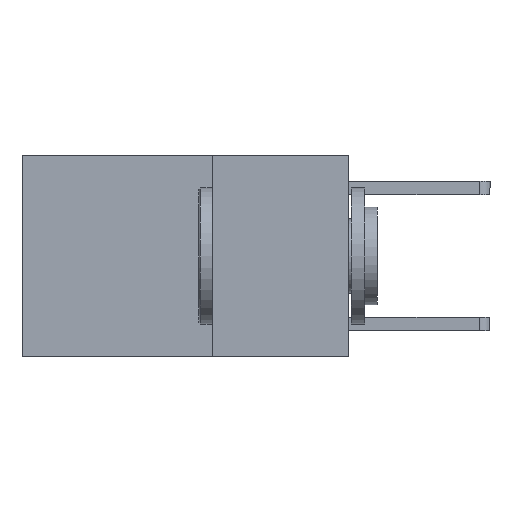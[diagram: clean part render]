
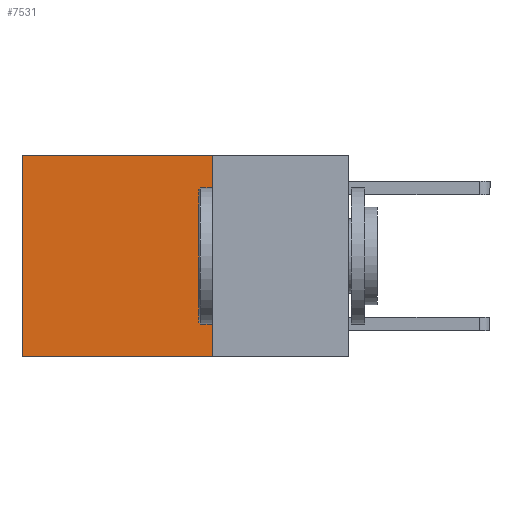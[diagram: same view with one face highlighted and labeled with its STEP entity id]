
A CAD part, left-side view. The second image highlights one B-rep face of the part: STEP entity #7531.
In plain terms, the highlighted planar face has unit normal (-1, 0, 0).
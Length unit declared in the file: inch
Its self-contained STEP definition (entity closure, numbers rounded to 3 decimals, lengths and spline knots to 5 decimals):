
#411 = EDGE_LOOP ( 'NONE', ( #4939, #6065, #1197, #7677 ) ) ;
#567 = PLANE ( 'NONE',  #1010 ) ;
#927 = VERTEX_POINT ( 'NONE', #7669 ) ;
#1010 = AXIS2_PLACEMENT_3D ( 'NONE', #4209, #9289, #8355 ) ;
#1098 = LINE ( 'NONE', #1873, #3606 ) ;
#1111 = VECTOR ( 'NONE', #6720, 39.37008 ) ;
#1197 = ORIENTED_EDGE ( 'NONE', *, *, #2684, .F. ) ;
#1653 = VERTEX_POINT ( 'NONE', #7351 ) ;
#1873 = CARTESIAN_POINT ( 'NONE',  ( 0.2625, 0.25, 0. ) ) ;
#1903 = VERTEX_POINT ( 'NONE', #5419 ) ;
#1950 = VECTOR ( 'NONE', #5726, 39.37008 ) ;
#2103 = CARTESIAN_POINT ( 'NONE',  ( 0.2625, 0.25, -0.37 ) ) ;
#2136 = EDGE_CURVE ( 'NONE', #1653, #927, #4411, .T. ) ;
#2684 = EDGE_CURVE ( 'NONE', #5913, #1903, #6620, .T. ) ;
#3606 = VECTOR ( 'NONE', #7428, 39.37008 ) ;
#4209 = CARTESIAN_POINT ( 'NONE',  ( 0.2625, 0.25, 0. ) ) ;
#4312 = CARTESIAN_POINT ( 'NONE',  ( 0.2625, 0.6, 0. ) ) ;
#4411 = LINE ( 'NONE', #4312, #8078 ) ;
#4884 = LINE ( 'NONE', #2103, #1950 ) ;
#4939 = ORIENTED_EDGE ( 'NONE', *, *, #2136, .T. ) ;
#5419 = CARTESIAN_POINT ( 'NONE',  ( 0.2625, 0.25, -0.37 ) ) ;
#5726 = DIRECTION ( 'NONE',  ( 0., 1., 0. ) ) ;
#5913 = VERTEX_POINT ( 'NONE', #7318 ) ;
#6013 = CARTESIAN_POINT ( 'NONE',  ( 0.2625, 0.25, 0. ) ) ;
#6065 = ORIENTED_EDGE ( 'NONE', *, *, #8498, .F. ) ;
#6620 = LINE ( 'NONE', #6013, #1111 ) ;
#6720 = DIRECTION ( 'NONE',  ( 0., 0., -1. ) ) ;
#7318 = CARTESIAN_POINT ( 'NONE',  ( 0.2625, 0.25, 0. ) ) ;
#7351 = CARTESIAN_POINT ( 'NONE',  ( 0.2625, 0.6, 0. ) ) ;
#7428 = DIRECTION ( 'NONE',  ( 0., 1., 0. ) ) ;
#7531 = ADVANCED_FACE ( 'NONE', ( #7815 ), #567, .F. ) ;
#7669 = CARTESIAN_POINT ( 'NONE',  ( 0.2625, 0.6, -0.37 ) ) ;
#7677 = ORIENTED_EDGE ( 'NONE', *, *, #8314, .T. ) ;
#7815 = FACE_OUTER_BOUND ( 'NONE', #411, .T. ) ;
#7975 = DIRECTION ( 'NONE',  ( 0., 0., -1. ) ) ;
#8078 = VECTOR ( 'NONE', #7975, 39.37008 ) ;
#8314 = EDGE_CURVE ( 'NONE', #5913, #1653, #1098, .T. ) ;
#8355 = DIRECTION ( 'NONE',  ( 0., 0., -1. ) ) ;
#8498 = EDGE_CURVE ( 'NONE', #1903, #927, #4884, .T. ) ;
#9289 = DIRECTION ( 'NONE',  ( 1., 0., 0. ) ) ;
